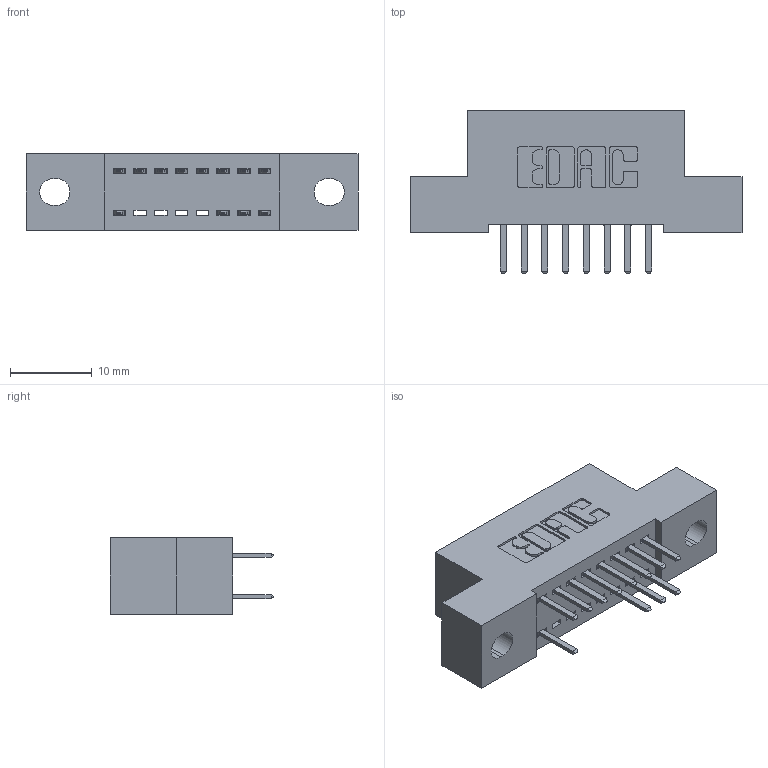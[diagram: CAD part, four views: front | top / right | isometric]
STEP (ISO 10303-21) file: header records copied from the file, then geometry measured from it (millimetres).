
FILE_DESCRIPTION (( 'STEP AP203' ), '1' );
FILE_NAME ('392-016-520-202.STEP', '2018-08-15T01:23:49', ( '' ), ( '' ), 'SwSTEP 2.0', 'SolidWorks 2016', '' );
FILE_SCHEMA (( 'CONFIG_CONTROL_DESIGN' ));
Length unit declared in the file: inch
Products named in the file (3): 342 Part_.128 Slot; 345-292-001_345-293-120; 392-016-520-202
Assembly tree (13 placements, depth 2):
  392-016-520-202
    342 Part_.128 Slot
    345-292-001_345-293-120  x12
Bounding box: 40.64 x 20.02 x 9.4 mm (x, y, z)
Volume: 3397.2 mm3; surface area: 4240 mm2
Topology: 13 solids, 13 shells, 810 faces, 2351 edges, 1534 vertices
Faces by surface type: plane 550, cylinder 260
Entity records: 9533 total; most frequent: CARTESIAN_POINT 1650, ORIENTED_EDGE 1578, DIRECTION 1453, EDGE_CURVE 789, VECTOR 657, LINE 657, VERTEX_POINT 522, AXIS2_PLACEMENT_3D 398
